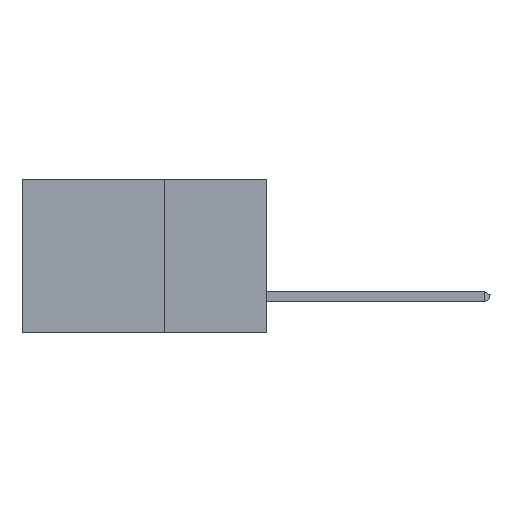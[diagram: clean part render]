
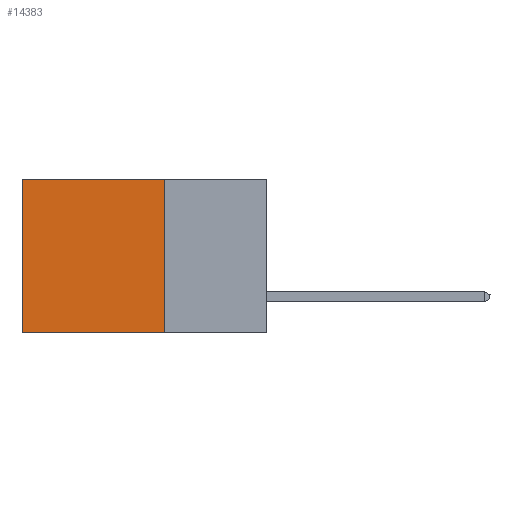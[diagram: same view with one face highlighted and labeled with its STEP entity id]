
A CAD part, left-side view. The second image highlights one B-rep face of the part: STEP entity #14383.
In plain terms, the highlighted planar face has unit normal (-1, 0, 0).
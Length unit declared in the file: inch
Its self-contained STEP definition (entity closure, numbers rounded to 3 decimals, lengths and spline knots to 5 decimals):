
#118 = DIRECTION ( 'NONE',  ( 0., 0., -1. ) ) ;
#680 = VERTEX_POINT ( 'NONE', #5559 ) ;
#1341 = VERTEX_POINT ( 'NONE', #7928 ) ;
#1487 = ORIENTED_EDGE ( 'NONE', *, *, #7828, .T. ) ;
#2440 = ORIENTED_EDGE ( 'NONE', *, *, #4368, .F. ) ;
#2645 = LINE ( 'NONE', #14479, #11563 ) ;
#2973 = DIRECTION ( 'NONE',  ( 1., 0., 0. ) ) ;
#4177 = VERTEX_POINT ( 'NONE', #9591 ) ;
#4368 = EDGE_CURVE ( 'NONE', #4177, #1341, #5285, .T. ) ;
#4718 = VECTOR ( 'NONE', #9375, 39.37008 ) ;
#4756 = EDGE_CURVE ( 'NONE', #680, #14962, #9250, .T. ) ;
#4981 = EDGE_LOOP ( 'NONE', ( #1487, #2440, #12767, #6771 ) ) ;
#5082 = PLANE ( 'NONE',  #12156 ) ;
#5279 = CARTESIAN_POINT ( 'NONE',  ( 0.2875, 0.25, -0.375 ) ) ;
#5285 = LINE ( 'NONE', #12103, #9638 ) ;
#5440 = DIRECTION ( 'NONE',  ( 0., 0., -1. ) ) ;
#5559 = CARTESIAN_POINT ( 'NONE',  ( 0.2875, 0.25, 0. ) ) ;
#5975 = CARTESIAN_POINT ( 'NONE',  ( 0.2875, 0.25, 0. ) ) ;
#6254 = DIRECTION ( 'NONE',  ( 0., 1., 0. ) ) ;
#6771 = ORIENTED_EDGE ( 'NONE', *, *, #4756, .T. ) ;
#7155 = CARTESIAN_POINT ( 'NONE',  ( 0.2875, 0.25, -0.375 ) ) ;
#7828 = EDGE_CURVE ( 'NONE', #14962, #1341, #2645, .T. ) ;
#7901 = LINE ( 'NONE', #7155, #12467 ) ;
#7928 = CARTESIAN_POINT ( 'NONE',  ( 0.2875, 0.6, -0.375 ) ) ;
#8337 = FACE_OUTER_BOUND ( 'NONE', #4981, .T. ) ;
#9250 = LINE ( 'NONE', #5975, #4718 ) ;
#9375 = DIRECTION ( 'NONE',  ( 0., 1., 0. ) ) ;
#9591 = CARTESIAN_POINT ( 'NONE',  ( 0.2875, 0.25, -0.375 ) ) ;
#9638 = VECTOR ( 'NONE', #6254, 39.37008 ) ;
#9700 = DIRECTION ( 'NONE',  ( 0., 0., -1. ) ) ;
#10693 = EDGE_CURVE ( 'NONE', #680, #4177, #7901, .T. ) ;
#11563 = VECTOR ( 'NONE', #9700, 39.37008 ) ;
#12103 = CARTESIAN_POINT ( 'NONE',  ( 0.2875, 0.25, -0.375 ) ) ;
#12156 = AXIS2_PLACEMENT_3D ( 'NONE', #5279, #2973, #5440 ) ;
#12288 = CARTESIAN_POINT ( 'NONE',  ( 0.2875, 0.6, 0. ) ) ;
#12467 = VECTOR ( 'NONE', #118, 39.37008 ) ;
#12767 = ORIENTED_EDGE ( 'NONE', *, *, #10693, .F. ) ;
#14383 = ADVANCED_FACE ( 'NONE', ( #8337 ), #5082, .F. ) ;
#14479 = CARTESIAN_POINT ( 'NONE',  ( 0.2875, 0.6, -0.375 ) ) ;
#14962 = VERTEX_POINT ( 'NONE', #12288 ) ;
